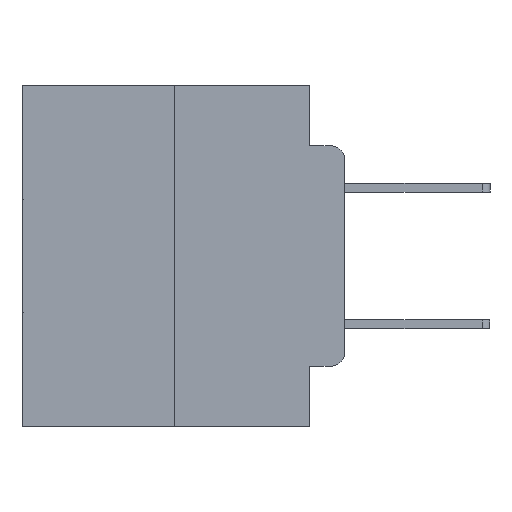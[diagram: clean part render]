
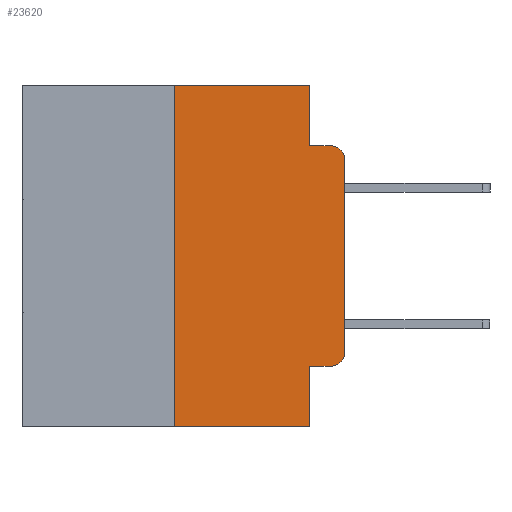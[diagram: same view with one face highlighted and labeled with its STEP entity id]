
A CAD part, left-side view. The second image highlights one B-rep face of the part: STEP entity #23620.
In plain terms, the highlighted planar face has unit normal (-1, 0, 0).
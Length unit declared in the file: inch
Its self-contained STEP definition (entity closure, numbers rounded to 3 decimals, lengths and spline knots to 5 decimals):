
#79 = DIRECTION ( 'NONE',  ( 0., -1., 0. ) ) ;
#172 = VERTEX_POINT ( 'NONE', #14135 ) ;
#320 = VERTEX_POINT ( 'NONE', #18706 ) ;
#1266 = VECTOR ( 'NONE', #27496, 39.37008 ) ;
#1604 = FACE_OUTER_BOUND ( 'NONE', #10223, .T. ) ;
#2114 = AXIS2_PLACEMENT_3D ( 'NONE', #25095, #12472, #27192 ) ;
#2319 = VECTOR ( 'NONE', #10166, 39.37008 ) ;
#2435 = ORIENTED_EDGE ( 'NONE', *, *, #15729, .T. ) ;
#2441 = VECTOR ( 'NONE', #19287, 39.37008 ) ;
#2563 = CIRCLE ( 'NONE', #24631, 0.02 ) ;
#2575 = VECTOR ( 'NONE', #3250, 39.37008 ) ;
#2704 = EDGE_CURVE ( 'NONE', #18584, #23072, #3125, .T. ) ;
#3125 = LINE ( 'NONE', #18678, #2441 ) ;
#3134 = VECTOR ( 'NONE', #7051, 39.37008 ) ;
#3250 = DIRECTION ( 'NONE',  ( 0., 0., -1. ) ) ;
#3459 = ORIENTED_EDGE ( 'NONE', *, *, #4196, .F. ) ;
#3680 = VERTEX_POINT ( 'NONE', #23167 ) ;
#3833 = ORIENTED_EDGE ( 'NONE', *, *, #2704, .T. ) ;
#4196 = EDGE_CURVE ( 'NONE', #14837, #8141, #6138, .T. ) ;
#5460 = CARTESIAN_POINT ( 'NONE',  ( 0., 0.051, 0. ) ) ;
#5647 = EDGE_CURVE ( 'NONE', #14850, #14837, #25273, .T. ) ;
#5840 = CARTESIAN_POINT ( 'NONE',  ( 0., 0.051, -0.4115 ) ) ;
#6138 = LINE ( 'NONE', #24409, #16861 ) ;
#7051 = DIRECTION ( 'NONE',  ( 0., 0., -1. ) ) ;
#7941 = VECTOR ( 'NONE', #25593, 39.37008 ) ;
#8141 = VERTEX_POINT ( 'NONE', #20680 ) ;
#8367 = EDGE_CURVE ( 'NONE', #13512, #14850, #13645, .T. ) ;
#8566 = EDGE_CURVE ( 'NONE', #3680, #320, #20248, .T. ) ;
#8820 = LINE ( 'NONE', #5840, #2319 ) ;
#8834 = DIRECTION ( 'NONE',  ( 1., 0., 0. ) ) ;
#8968 = CARTESIAN_POINT ( 'NONE',  ( 0., 0.051, -0.0885 ) ) ;
#9992 = EDGE_CURVE ( 'NONE', #17026, #13512, #27702, .T. ) ;
#10166 = DIRECTION ( 'NONE',  ( 0., -1., 0. ) ) ;
#10223 = EDGE_LOOP ( 'NONE', ( #3833, #11586, #3459, #27392, #20897, #16604, #11918, #18912, #17589, #2435 ) ) ;
#10923 = CARTESIAN_POINT ( 'NONE',  ( 0., 0.02, -0.1085 ) ) ;
#11417 = EDGE_CURVE ( 'NONE', #3680, #172, #8820, .T. ) ;
#11586 = ORIENTED_EDGE ( 'NONE', *, *, #24688, .T. ) ;
#11918 = ORIENTED_EDGE ( 'NONE', *, *, #22948, .T. ) ;
#12151 = DIRECTION ( 'NONE',  ( 0., 0., 1. ) ) ;
#12472 = DIRECTION ( 'NONE',  ( -1., 0., 0. ) ) ;
#12702 = CARTESIAN_POINT ( 'NONE',  ( 0., 0., -0.3915 ) ) ;
#13086 = DIRECTION ( 'NONE',  ( 0., 0., -1. ) ) ;
#13512 = VERTEX_POINT ( 'NONE', #17335 ) ;
#13517 = AXIS2_PLACEMENT_3D ( 'NONE', #19445, #8834, #23661 ) ;
#13519 = LINE ( 'NONE', #23332, #1266 ) ;
#13645 = LINE ( 'NONE', #17168, #7941 ) ;
#13688 = CIRCLE ( 'NONE', #2114, 0.02 ) ;
#14135 = CARTESIAN_POINT ( 'NONE',  ( 0., 0.02, -0.4115 ) ) ;
#14837 = VERTEX_POINT ( 'NONE', #8968 ) ;
#14850 = VERTEX_POINT ( 'NONE', #21792 ) ;
#15729 = EDGE_CURVE ( 'NONE', #172, #18584, #13688, .T. ) ;
#16604 = ORIENTED_EDGE ( 'NONE', *, *, #9992, .F. ) ;
#16861 = VECTOR ( 'NONE', #79, 39.37008 ) ;
#17026 = VERTEX_POINT ( 'NONE', #18258 ) ;
#17168 = CARTESIAN_POINT ( 'NONE',  ( 0., 0.473, 0. ) ) ;
#17331 = PLANE ( 'NONE',  #13517 ) ;
#17335 = CARTESIAN_POINT ( 'NONE',  ( 0., 0.25, 0. ) ) ;
#17589 = ORIENTED_EDGE ( 'NONE', *, *, #11417, .T. ) ;
#18258 = CARTESIAN_POINT ( 'NONE',  ( 0., 0.25, -0.5 ) ) ;
#18584 = VERTEX_POINT ( 'NONE', #12702 ) ;
#18678 = CARTESIAN_POINT ( 'NONE',  ( 0., 0., 0. ) ) ;
#18706 = CARTESIAN_POINT ( 'NONE',  ( 0., 0.051, -0.5 ) ) ;
#18912 = ORIENTED_EDGE ( 'NONE', *, *, #8566, .F. ) ;
#19287 = DIRECTION ( 'NONE',  ( 0., 0., 1. ) ) ;
#19445 = CARTESIAN_POINT ( 'NONE',  ( 0., 0.473, 0. ) ) ;
#19664 = CARTESIAN_POINT ( 'NONE',  ( 0., 0., -0.1085 ) ) ;
#19838 = CARTESIAN_POINT ( 'NONE',  ( 0., 0.051, 0. ) ) ;
#20248 = LINE ( 'NONE', #19838, #3134 ) ;
#20680 = CARTESIAN_POINT ( 'NONE',  ( 0., 0.02, -0.0885 ) ) ;
#20897 = ORIENTED_EDGE ( 'NONE', *, *, #8367, .F. ) ;
#21792 = CARTESIAN_POINT ( 'NONE',  ( 0., 0.051, 0. ) ) ;
#22845 = VECTOR ( 'NONE', #12151, 39.37008 ) ;
#22948 = EDGE_CURVE ( 'NONE', #17026, #320, #13519, .T. ) ;
#23072 = VERTEX_POINT ( 'NONE', #19664 ) ;
#23167 = CARTESIAN_POINT ( 'NONE',  ( 0., 0.051, -0.4115 ) ) ;
#23332 = CARTESIAN_POINT ( 'NONE',  ( 0., 0.473, -0.5 ) ) ;
#23620 = ADVANCED_FACE ( 'NONE', ( #1604 ), #17331, .F. ) ;
#23661 = DIRECTION ( 'NONE',  ( 0., 0., -1. ) ) ;
#24409 = CARTESIAN_POINT ( 'NONE',  ( 0., 0.051, -0.0885 ) ) ;
#24631 = AXIS2_PLACEMENT_3D ( 'NONE', #10923, #25699, #13086 ) ;
#24688 = EDGE_CURVE ( 'NONE', #23072, #8141, #2563, .T. ) ;
#24778 = CARTESIAN_POINT ( 'NONE',  ( 0., 0.25, 0. ) ) ;
#25095 = CARTESIAN_POINT ( 'NONE',  ( 0., 0.02, -0.3915 ) ) ;
#25273 = LINE ( 'NONE', #5460, #2575 ) ;
#25593 = DIRECTION ( 'NONE',  ( 0., -1., 0. ) ) ;
#25699 = DIRECTION ( 'NONE',  ( -1., 0., 0. ) ) ;
#27192 = DIRECTION ( 'NONE',  ( 0., 0., -1. ) ) ;
#27392 = ORIENTED_EDGE ( 'NONE', *, *, #5647, .F. ) ;
#27496 = DIRECTION ( 'NONE',  ( 0., -1., 0. ) ) ;
#27702 = LINE ( 'NONE', #24778, #22845 ) ;
